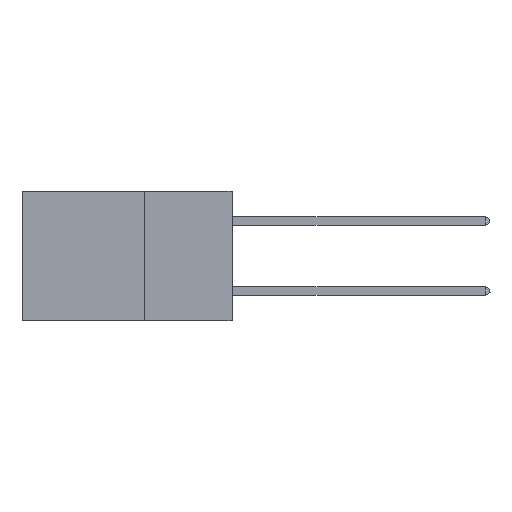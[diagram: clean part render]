
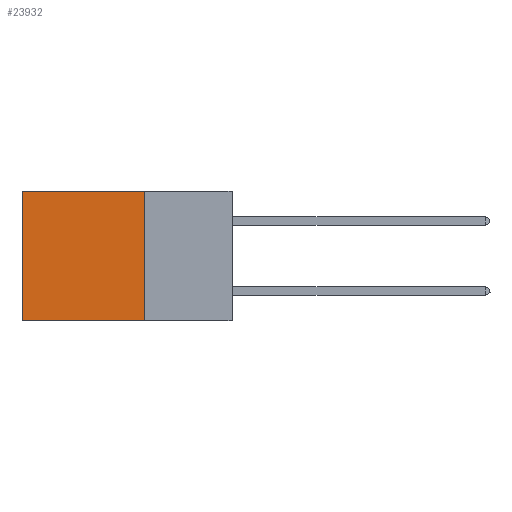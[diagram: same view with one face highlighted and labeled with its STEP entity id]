
A CAD part, left-side view. The second image highlights one B-rep face of the part: STEP entity #23932.
In plain terms, the highlighted planar face has unit normal (-1, 0, 0).
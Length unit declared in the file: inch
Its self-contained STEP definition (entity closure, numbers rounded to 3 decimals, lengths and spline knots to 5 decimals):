
#21 = FACE_OUTER_BOUND ( 'NONE', #1549, .T. ) ;
#118 = ORIENTED_EDGE ( 'NONE', *, *, #22811, .F. ) ;
#1549 = EDGE_LOOP ( 'NONE', ( #2257, #118, #1793, #8050 ) ) ;
#1793 = ORIENTED_EDGE ( 'NONE', *, *, #2809, .F. ) ;
#2070 = DIRECTION ( 'NONE',  ( 0., 0., -1. ) ) ;
#2257 = ORIENTED_EDGE ( 'NONE', *, *, #11060, .T. ) ;
#2809 = EDGE_CURVE ( 'NONE', #10023, #11113, #23411, .T. ) ;
#3136 = CARTESIAN_POINT ( 'NONE',  ( 0.2875, 0.6, 0. ) ) ;
#3483 = DIRECTION ( 'NONE',  ( 1., 0., 0. ) ) ;
#4519 = LINE ( 'NONE', #24815, #8004 ) ;
#4978 = CARTESIAN_POINT ( 'NONE',  ( 0.2875, 0.25, 0. ) ) ;
#6344 = DIRECTION ( 'NONE',  ( 0., 1., 0. ) ) ;
#6834 = AXIS2_PLACEMENT_3D ( 'NONE', #22516, #3483, #2070 ) ;
#7114 = LINE ( 'NONE', #4978, #9343 ) ;
#7124 = VECTOR ( 'NONE', #17921, 39.37008 ) ;
#8004 = VECTOR ( 'NONE', #6344, 39.37008 ) ;
#8050 = ORIENTED_EDGE ( 'NONE', *, *, #12430, .T. ) ;
#9343 = VECTOR ( 'NONE', #10939, 39.37008 ) ;
#9851 = DIRECTION ( 'NONE',  ( 0., 0., -1. ) ) ;
#10023 = VERTEX_POINT ( 'NONE', #20929 ) ;
#10939 = DIRECTION ( 'NONE',  ( 0., 1., 0. ) ) ;
#11060 = EDGE_CURVE ( 'NONE', #23730, #21407, #25701, .T. ) ;
#11113 = VERTEX_POINT ( 'NONE', #23166 ) ;
#12049 = CARTESIAN_POINT ( 'NONE',  ( 0.2875, 0.6, 0. ) ) ;
#12430 = EDGE_CURVE ( 'NONE', #10023, #23730, #7114, .T. ) ;
#13569 = CARTESIAN_POINT ( 'NONE',  ( 0.2875, 0.25, 0. ) ) ;
#17921 = DIRECTION ( 'NONE',  ( 0., 0., -1. ) ) ;
#18067 = VECTOR ( 'NONE', #9851, 39.37008 ) ;
#18629 = CARTESIAN_POINT ( 'NONE',  ( 0.2875, 0.6, -0.37 ) ) ;
#20470 = PLANE ( 'NONE',  #6834 ) ;
#20929 = CARTESIAN_POINT ( 'NONE',  ( 0.2875, 0.25, 0. ) ) ;
#21407 = VERTEX_POINT ( 'NONE', #18629 ) ;
#22516 = CARTESIAN_POINT ( 'NONE',  ( 0.2875, 0.25, 0. ) ) ;
#22811 = EDGE_CURVE ( 'NONE', #11113, #21407, #4519, .T. ) ;
#23166 = CARTESIAN_POINT ( 'NONE',  ( 0.2875, 0.25, -0.37 ) ) ;
#23411 = LINE ( 'NONE', #13569, #7124 ) ;
#23730 = VERTEX_POINT ( 'NONE', #3136 ) ;
#23932 = ADVANCED_FACE ( 'NONE', ( #21 ), #20470, .F. ) ;
#24815 = CARTESIAN_POINT ( 'NONE',  ( 0.2875, 0.25, -0.37 ) ) ;
#25701 = LINE ( 'NONE', #12049, #18067 ) ;
